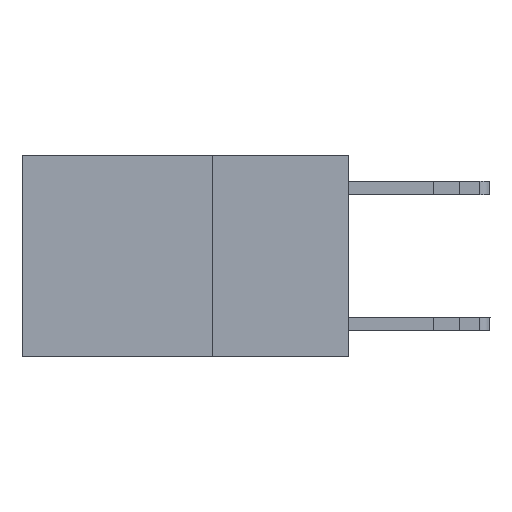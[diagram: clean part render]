
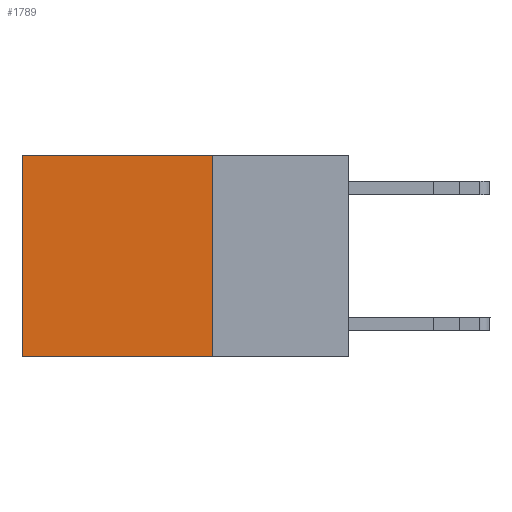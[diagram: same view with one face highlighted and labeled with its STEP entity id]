
A CAD part, left-side view. The second image highlights one B-rep face of the part: STEP entity #1789.
In plain terms, the highlighted planar face has unit normal (-1, 0, 0).
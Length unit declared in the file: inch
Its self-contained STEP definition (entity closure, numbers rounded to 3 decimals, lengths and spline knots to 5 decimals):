
#708 = DIRECTION ( 'NONE',  ( 0., 0., -1. ) ) ;
#1172 = VECTOR ( 'NONE', #17036, 39.37008 ) ;
#1272 = ORIENTED_EDGE ( 'NONE', *, *, #7376, .T. ) ;
#1564 = EDGE_CURVE ( 'NONE', #5524, #2183, #13895, .T. ) ;
#1591 = LINE ( 'NONE', #17913, #1172 ) ;
#1789 = ADVANCED_FACE ( 'NONE', ( #14956 ), #15571, .F. ) ;
#2183 = VERTEX_POINT ( 'NONE', #19722 ) ;
#2679 = CARTESIAN_POINT ( 'NONE',  ( 0.2625, 0.25, 0. ) ) ;
#4082 = EDGE_LOOP ( 'NONE', ( #6394, #11440, #17254, #1272 ) ) ;
#5104 = CARTESIAN_POINT ( 'NONE',  ( 0.2625, 0.6, 0. ) ) ;
#5384 = DIRECTION ( 'NONE',  ( 0., 0., -1. ) ) ;
#5483 = VECTOR ( 'NONE', #5384, 39.37008 ) ;
#5524 = VERTEX_POINT ( 'NONE', #2679 ) ;
#5844 = CARTESIAN_POINT ( 'NONE',  ( 0.2625, 0.6, 0. ) ) ;
#5875 = CARTESIAN_POINT ( 'NONE',  ( 0.2625, 0.25, 0. ) ) ;
#6394 = ORIENTED_EDGE ( 'NONE', *, *, #17085, .T. ) ;
#7044 = CARTESIAN_POINT ( 'NONE',  ( 0.2625, 0.6, -0.37 ) ) ;
#7376 = EDGE_CURVE ( 'NONE', #5524, #7758, #8558, .T. ) ;
#7758 = VERTEX_POINT ( 'NONE', #5104 ) ;
#8410 = VECTOR ( 'NONE', #13316, 39.37008 ) ;
#8558 = LINE ( 'NONE', #13755, #8410 ) ;
#8972 = LINE ( 'NONE', #5844, #5483 ) ;
#9551 = EDGE_CURVE ( 'NONE', #2183, #9823, #1591, .T. ) ;
#9823 = VERTEX_POINT ( 'NONE', #7044 ) ;
#10967 = AXIS2_PLACEMENT_3D ( 'NONE', #16029, #14368, #14295 ) ;
#11440 = ORIENTED_EDGE ( 'NONE', *, *, #9551, .F. ) ;
#11904 = VECTOR ( 'NONE', #708, 39.37008 ) ;
#13316 = DIRECTION ( 'NONE',  ( 0., 1., 0. ) ) ;
#13755 = CARTESIAN_POINT ( 'NONE',  ( 0.2625, 0.25, 0. ) ) ;
#13895 = LINE ( 'NONE', #5875, #11904 ) ;
#14295 = DIRECTION ( 'NONE',  ( 0., 0., -1. ) ) ;
#14368 = DIRECTION ( 'NONE',  ( 1., 0., 0. ) ) ;
#14956 = FACE_OUTER_BOUND ( 'NONE', #4082, .T. ) ;
#15571 = PLANE ( 'NONE',  #10967 ) ;
#16029 = CARTESIAN_POINT ( 'NONE',  ( 0.2625, 0.25, 0. ) ) ;
#17036 = DIRECTION ( 'NONE',  ( 0., 1., 0. ) ) ;
#17085 = EDGE_CURVE ( 'NONE', #7758, #9823, #8972, .T. ) ;
#17254 = ORIENTED_EDGE ( 'NONE', *, *, #1564, .F. ) ;
#17913 = CARTESIAN_POINT ( 'NONE',  ( 0.2625, 0.25, -0.37 ) ) ;
#19722 = CARTESIAN_POINT ( 'NONE',  ( 0.2625, 0.25, -0.37 ) ) ;
